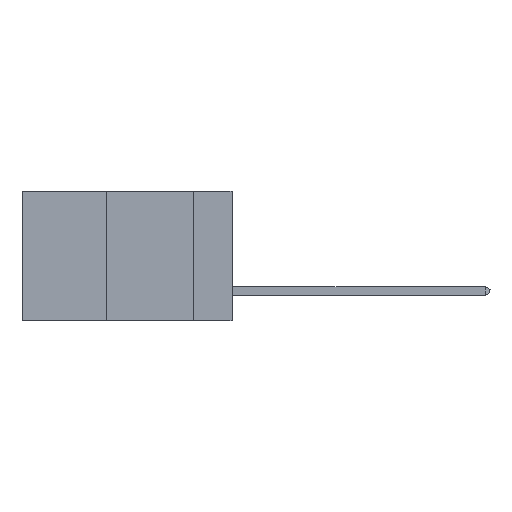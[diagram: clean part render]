
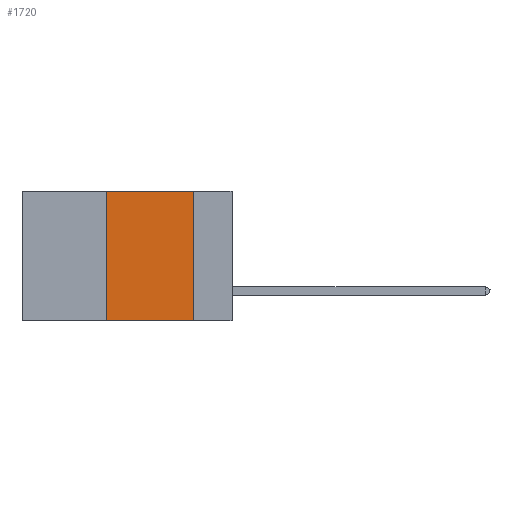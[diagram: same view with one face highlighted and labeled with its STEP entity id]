
A CAD part, left-side view. The second image highlights one B-rep face of the part: STEP entity #1720.
In plain terms, the highlighted planar face has unit normal (-1, 0, 0).
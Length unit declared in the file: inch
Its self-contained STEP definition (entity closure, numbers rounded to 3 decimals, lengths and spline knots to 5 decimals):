
#574 = VERTEX_POINT ( 'NONE', #13379 ) ;
#1492 = DIRECTION ( 'NONE',  ( 0., 0., -1. ) ) ;
#1511 = CARTESIAN_POINT ( 'NONE',  ( 0., 0.36, -0.37 ) ) ;
#1707 = VECTOR ( 'NONE', #11849, 39.37008 ) ;
#1720 = ADVANCED_FACE ( 'NONE', ( #26299 ), #4178, .F. ) ;
#3815 = LINE ( 'NONE', #17093, #20118 ) ;
#4178 = PLANE ( 'NONE',  #17939 ) ;
#8339 = EDGE_CURVE ( 'NONE', #33737, #574, #14862, .T. ) ;
#8410 = LINE ( 'NONE', #11963, #1707 ) ;
#9881 = DIRECTION ( 'NONE',  ( 0., 0., 1. ) ) ;
#11776 = CARTESIAN_POINT ( 'NONE',  ( 0., 0.11, 0. ) ) ;
#11849 = DIRECTION ( 'NONE',  ( 0., 0., -1. ) ) ;
#11963 = CARTESIAN_POINT ( 'NONE',  ( 0., 0.11, 0. ) ) ;
#12088 = EDGE_CURVE ( 'NONE', #574, #30571, #3815, .T. ) ;
#12748 = DIRECTION ( 'NONE',  ( 1., 0., 0. ) ) ;
#13379 = CARTESIAN_POINT ( 'NONE',  ( 0., 0.36, 0. ) ) ;
#14862 = LINE ( 'NONE', #25153, #26100 ) ;
#16668 = EDGE_CURVE ( 'NONE', #33737, #23648, #29755, .T. ) ;
#17066 = EDGE_CURVE ( 'NONE', #30571, #23648, #8410, .T. ) ;
#17093 = CARTESIAN_POINT ( 'NONE',  ( 0., 0.6, 0. ) ) ;
#17939 = AXIS2_PLACEMENT_3D ( 'NONE', #25869, #12748, #1492 ) ;
#20118 = VECTOR ( 'NONE', #33365, 39.37008 ) ;
#22287 = ORIENTED_EDGE ( 'NONE', *, *, #8339, .F. ) ;
#23648 = VERTEX_POINT ( 'NONE', #26334 ) ;
#24470 = ORIENTED_EDGE ( 'NONE', *, *, #17066, .F. ) ;
#24703 = VECTOR ( 'NONE', #26715, 39.37008 ) ;
#25107 = ORIENTED_EDGE ( 'NONE', *, *, #16668, .T. ) ;
#25153 = CARTESIAN_POINT ( 'NONE',  ( 0., 0.36, 0. ) ) ;
#25869 = CARTESIAN_POINT ( 'NONE',  ( 0., 0.6, 0. ) ) ;
#26100 = VECTOR ( 'NONE', #9881, 39.37008 ) ;
#26288 = EDGE_LOOP ( 'NONE', ( #24470, #29905, #22287, #25107 ) ) ;
#26299 = FACE_OUTER_BOUND ( 'NONE', #26288, .T. ) ;
#26334 = CARTESIAN_POINT ( 'NONE',  ( 0., 0.11, -0.37 ) ) ;
#26715 = DIRECTION ( 'NONE',  ( 0., -1., 0. ) ) ;
#29755 = LINE ( 'NONE', #31903, #24703 ) ;
#29905 = ORIENTED_EDGE ( 'NONE', *, *, #12088, .F. ) ;
#30571 = VERTEX_POINT ( 'NONE', #11776 ) ;
#31903 = CARTESIAN_POINT ( 'NONE',  ( 0., 0.6, -0.37 ) ) ;
#33365 = DIRECTION ( 'NONE',  ( 0., -1., 0. ) ) ;
#33737 = VERTEX_POINT ( 'NONE', #1511 ) ;
